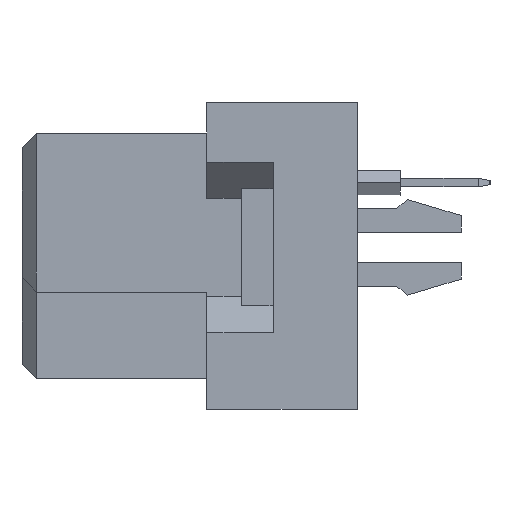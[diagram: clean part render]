
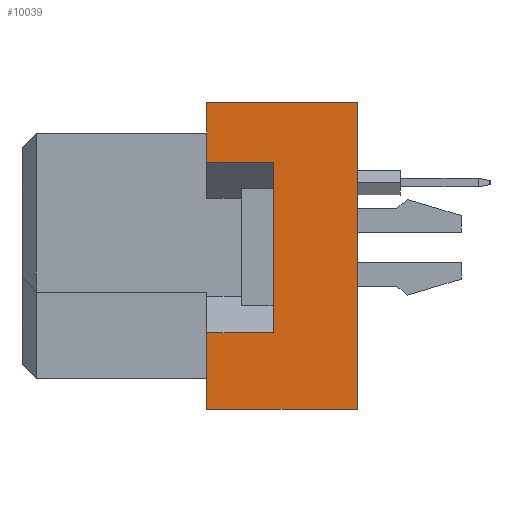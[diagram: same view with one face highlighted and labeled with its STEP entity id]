
A CAD part, left-side view. The second image highlights one B-rep face of the part: STEP entity #10039.
In plain terms, the highlighted planar face has unit normal (-1, 0, 0).
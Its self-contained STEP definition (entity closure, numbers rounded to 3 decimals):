
#373 = DIRECTION ( 'NONE',  ( 0., 0., 1. ) ) ;
#810 = LINE ( 'NONE', #36443, #16799 ) ;
#998 = ORIENTED_EDGE ( 'NONE', *, *, #28016, .F. ) ;
#2608 = CARTESIAN_POINT ( 'NONE',  ( -47.5, -11.6, 5.3 ) ) ;
#4703 = CARTESIAN_POINT ( 'NONE',  ( -47.5, -11.6, -5.3 ) ) ;
#4818 = EDGE_CURVE ( 'NONE', #9794, #38627, #810, .T. ) ;
#5377 = EDGE_CURVE ( 'NONE', #10272, #18174, #16213, .T. ) ;
#6213 = VECTOR ( 'NONE', #35540, 1000. ) ;
#9446 = LINE ( 'NONE', #33567, #37014 ) ;
#9794 = VERTEX_POINT ( 'NONE', #22156 ) ;
#10039 = ADVANCED_FACE ( 'NONE', ( #30064 ), #24110, .T. ) ;
#10272 = VERTEX_POINT ( 'NONE', #4703 ) ;
#10818 = ORIENTED_EDGE ( 'NONE', *, *, #12085, .F. ) ;
#11230 = LINE ( 'NONE', #17352, #6213 ) ;
#11255 = LINE ( 'NONE', #23504, #38613 ) ;
#11882 = EDGE_CURVE ( 'NONE', #29621, #13629, #31304, .T. ) ;
#12085 = EDGE_CURVE ( 'NONE', #13629, #22321, #31728, .T. ) ;
#12137 = CARTESIAN_POINT ( 'NONE',  ( -47.5, -6.4, -5.3 ) ) ;
#12749 = CARTESIAN_POINT ( 'NONE',  ( -47.5, -8.7, 3.25 ) ) ;
#13629 = VERTEX_POINT ( 'NONE', #13886 ) ;
#13841 = ORIENTED_EDGE ( 'NONE', *, *, #28813, .F. ) ;
#13886 = CARTESIAN_POINT ( 'NONE',  ( -47.5, -6.4, 3.25 ) ) ;
#15732 = ORIENTED_EDGE ( 'NONE', *, *, #20413, .F. ) ;
#15888 = VECTOR ( 'NONE', #28758, 1000. ) ;
#16052 = LINE ( 'NONE', #24384, #23791 ) ;
#16213 = LINE ( 'NONE', #37178, #32523 ) ;
#16470 = CARTESIAN_POINT ( 'NONE',  ( -47.5, -8.7, 3.25 ) ) ;
#16799 = VECTOR ( 'NONE', #36245, 1000. ) ;
#16895 = CARTESIAN_POINT ( 'NONE',  ( -47.5, -6.4, -2.65 ) ) ;
#17352 = CARTESIAN_POINT ( 'NONE',  ( -47.5, -11.6, 5.3 ) ) ;
#17427 = ORIENTED_EDGE ( 'NONE', *, *, #32490, .T. ) ;
#18174 = VERTEX_POINT ( 'NONE', #2608 ) ;
#18194 = CARTESIAN_POINT ( 'NONE',  ( -47.5, -11.6, 5.3 ) ) ;
#18274 = DIRECTION ( 'NONE',  ( 0., 0., 1. ) ) ;
#19030 = VECTOR ( 'NONE', #37044, 1000. ) ;
#19079 = ORIENTED_EDGE ( 'NONE', *, *, #11882, .F. ) ;
#20413 = EDGE_CURVE ( 'NONE', #29929, #38627, #11255, .T. ) ;
#22156 = CARTESIAN_POINT ( 'NONE',  ( -47.5, -8.7, -2.65 ) ) ;
#22321 = VERTEX_POINT ( 'NONE', #27201 ) ;
#22424 = CARTESIAN_POINT ( 'NONE',  ( -47.5, -6.4, -5.3 ) ) ;
#22545 = DIRECTION ( 'NONE',  ( 0., 0., 1. ) ) ;
#23504 = CARTESIAN_POINT ( 'NONE',  ( -47.5, -6.4, -5.3 ) ) ;
#23791 = VECTOR ( 'NONE', #18274, 1000. ) ;
#24110 = PLANE ( 'NONE',  #26528 ) ;
#24384 = CARTESIAN_POINT ( 'NONE',  ( -47.5, -8.7, -2.65 ) ) ;
#24684 = DIRECTION ( 'NONE',  ( -1., 0., 0. ) ) ;
#26528 = AXIS2_PLACEMENT_3D ( 'NONE', #18194, #24684, #373 ) ;
#27060 = DIRECTION ( 'NONE',  ( 0., 0., 1. ) ) ;
#27201 = CARTESIAN_POINT ( 'NONE',  ( -47.5, -6.4, 5.3 ) ) ;
#28016 = EDGE_CURVE ( 'NONE', #10272, #29929, #9446, .T. ) ;
#28758 = DIRECTION ( 'NONE',  ( 0., 0., 1. ) ) ;
#28813 = EDGE_CURVE ( 'NONE', #9794, #29621, #16052, .T. ) ;
#29621 = VERTEX_POINT ( 'NONE', #12749 ) ;
#29929 = VERTEX_POINT ( 'NONE', #12137 ) ;
#30064 = FACE_OUTER_BOUND ( 'NONE', #35036, .T. ) ;
#31304 = LINE ( 'NONE', #16470, #19030 ) ;
#31728 = LINE ( 'NONE', #22424, #15888 ) ;
#32490 = EDGE_CURVE ( 'NONE', #18174, #22321, #11230, .T. ) ;
#32523 = VECTOR ( 'NONE', #22545, 1000. ) ;
#33567 = CARTESIAN_POINT ( 'NONE',  ( -47.5, -11.6, -5.3 ) ) ;
#35036 = EDGE_LOOP ( 'NONE', ( #36796, #15732, #998, #39054, #17427, #10818, #19079, #13841 ) ) ;
#35540 = DIRECTION ( 'NONE',  ( 0., 1., 0. ) ) ;
#36245 = DIRECTION ( 'NONE',  ( 0., 1., 0. ) ) ;
#36443 = CARTESIAN_POINT ( 'NONE',  ( -47.5, -8.7, -2.65 ) ) ;
#36725 = DIRECTION ( 'NONE',  ( 0., 1., 0. ) ) ;
#36796 = ORIENTED_EDGE ( 'NONE', *, *, #4818, .T. ) ;
#37014 = VECTOR ( 'NONE', #36725, 1000. ) ;
#37044 = DIRECTION ( 'NONE',  ( 0., 1., 0. ) ) ;
#37178 = CARTESIAN_POINT ( 'NONE',  ( -47.5, -11.6, 5.3 ) ) ;
#38613 = VECTOR ( 'NONE', #27060, 1000. ) ;
#38627 = VERTEX_POINT ( 'NONE', #16895 ) ;
#39054 = ORIENTED_EDGE ( 'NONE', *, *, #5377, .T. ) ;
